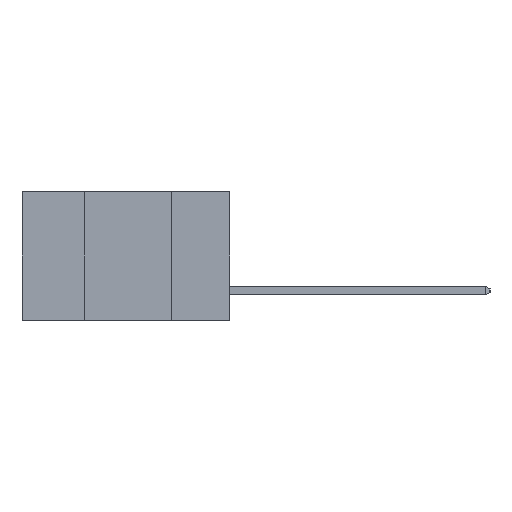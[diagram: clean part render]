
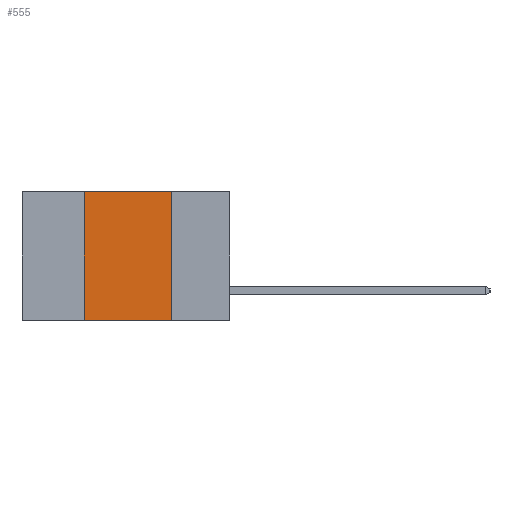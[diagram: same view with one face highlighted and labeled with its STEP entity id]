
A CAD part, left-side view. The second image highlights one B-rep face of the part: STEP entity #555.
In plain terms, the highlighted planar face has unit normal (-1, 0, 0).
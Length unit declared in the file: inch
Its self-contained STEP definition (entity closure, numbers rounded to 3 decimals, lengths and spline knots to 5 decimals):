
#320 = ORIENTED_EDGE ( 'NONE', *, *, #11596, .F. ) ;
#555 = ADVANCED_FACE ( 'NONE', ( #1551 ), #10408, .F. ) ;
#1551 = FACE_OUTER_BOUND ( 'NONE', #15229, .T. ) ;
#2277 = LINE ( 'NONE', #6473, #11243 ) ;
#3328 = CARTESIAN_POINT ( 'NONE',  ( 0., 0.42, 0. ) ) ;
#5087 = VECTOR ( 'NONE', #19664, 39.37008 ) ;
#5354 = LINE ( 'NONE', #16781, #6962 ) ;
#5811 = VERTEX_POINT ( 'NONE', #8520 ) ;
#6168 = VERTEX_POINT ( 'NONE', #3328 ) ;
#6473 = CARTESIAN_POINT ( 'NONE',  ( 0., 0.17, -0.37 ) ) ;
#6962 = VECTOR ( 'NONE', #21445, 39.37008 ) ;
#6990 = CARTESIAN_POINT ( 'NONE',  ( 0., 0.42, -0.37 ) ) ;
#7611 = DIRECTION ( 'NONE',  ( 0., 0., -1. ) ) ;
#7858 = VERTEX_POINT ( 'NONE', #6990 ) ;
#8066 = CARTESIAN_POINT ( 'NONE',  ( 0., 0.17, 0. ) ) ;
#8520 = CARTESIAN_POINT ( 'NONE',  ( 0., 0.17, -0.37 ) ) ;
#9171 = LINE ( 'NONE', #17904, #22695 ) ;
#9173 = EDGE_CURVE ( 'NONE', #7858, #5811, #5354, .T. ) ;
#9932 = AXIS2_PLACEMENT_3D ( 'NONE', #10594, #10928, #7611 ) ;
#10132 = DIRECTION ( 'NONE',  ( 0., 0., -1. ) ) ;
#10408 = PLANE ( 'NONE',  #9932 ) ;
#10594 = CARTESIAN_POINT ( 'NONE',  ( 0., 0.6, 0. ) ) ;
#10928 = DIRECTION ( 'NONE',  ( 1., 0., 0. ) ) ;
#11243 = VECTOR ( 'NONE', #10132, 39.37008 ) ;
#11596 = EDGE_CURVE ( 'NONE', #7858, #6168, #9171, .T. ) ;
#14061 = ORIENTED_EDGE ( 'NONE', *, *, #15285, .F. ) ;
#15229 = EDGE_LOOP ( 'NONE', ( #20163, #14061, #320, #18032 ) ) ;
#15285 = EDGE_CURVE ( 'NONE', #6168, #17799, #19418, .T. ) ;
#16501 = EDGE_CURVE ( 'NONE', #17799, #5811, #2277, .T. ) ;
#16781 = CARTESIAN_POINT ( 'NONE',  ( 0., 0.6, -0.37 ) ) ;
#17122 = DIRECTION ( 'NONE',  ( 0., 0., 1. ) ) ;
#17799 = VERTEX_POINT ( 'NONE', #8066 ) ;
#17904 = CARTESIAN_POINT ( 'NONE',  ( 0., 0.42, -0.37 ) ) ;
#18032 = ORIENTED_EDGE ( 'NONE', *, *, #9173, .T. ) ;
#19418 = LINE ( 'NONE', #20161, #5087 ) ;
#19664 = DIRECTION ( 'NONE',  ( 0., -1., 0. ) ) ;
#20161 = CARTESIAN_POINT ( 'NONE',  ( 0., 0.6, 0. ) ) ;
#20163 = ORIENTED_EDGE ( 'NONE', *, *, #16501, .F. ) ;
#21445 = DIRECTION ( 'NONE',  ( 0., -1., 0. ) ) ;
#22695 = VECTOR ( 'NONE', #17122, 39.37008 ) ;
